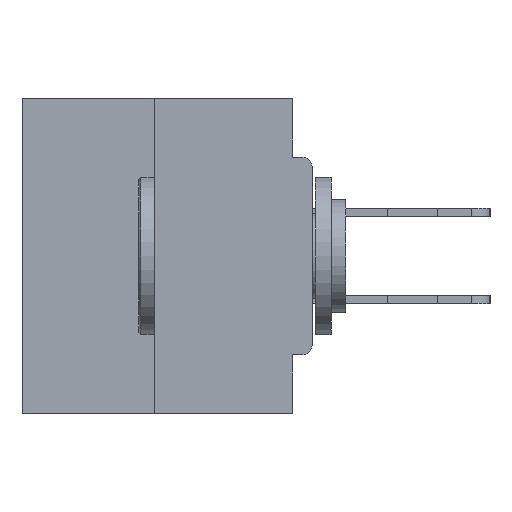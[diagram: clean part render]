
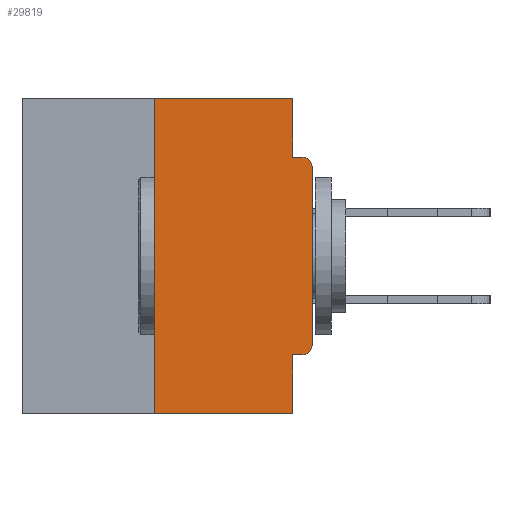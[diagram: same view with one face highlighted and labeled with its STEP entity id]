
A CAD part, left-side view. The second image highlights one B-rep face of the part: STEP entity #29819.
In plain terms, the highlighted planar face has unit normal (-1, 0, 0).
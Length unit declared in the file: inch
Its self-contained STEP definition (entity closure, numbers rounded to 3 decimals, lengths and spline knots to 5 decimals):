
#971 = CARTESIAN_POINT ( 'NONE',  ( 0., 0., -0.4065 ) ) ;
#1369 = DIRECTION ( 'NONE',  ( 0., -1., 0. ) ) ;
#1445 = CARTESIAN_POINT ( 'NONE',  ( 0., 0.031, 0. ) ) ;
#1737 = ORIENTED_EDGE ( 'NONE', *, *, #7454, .T. ) ;
#2048 = VERTEX_POINT ( 'NONE', #5673 ) ;
#2219 = ORIENTED_EDGE ( 'NONE', *, *, #28640, .F. ) ;
#2368 = VERTEX_POINT ( 'NONE', #9984 ) ;
#2789 = ORIENTED_EDGE ( 'NONE', *, *, #19677, .F. ) ;
#3756 = AXIS2_PLACEMENT_3D ( 'NONE', #20615, #26298, #30040 ) ;
#3862 = CARTESIAN_POINT ( 'NONE',  ( 0., 0., -0.1085 ) ) ;
#4383 = DIRECTION ( 'NONE',  ( 0., 0., 1. ) ) ;
#4483 = LINE ( 'NONE', #29040, #16997 ) ;
#4510 = CARTESIAN_POINT ( 'NONE',  ( 0., 0.25, 0. ) ) ;
#4665 = EDGE_CURVE ( 'NONE', #15509, #35964, #20862, .T. ) ;
#5628 = FACE_OUTER_BOUND ( 'NONE', #11698, .T. ) ;
#5673 = CARTESIAN_POINT ( 'NONE',  ( 0., 0., -0.3915 ) ) ;
#6299 = CARTESIAN_POINT ( 'NONE',  ( 0., 0.46, -0.5 ) ) ;
#6460 = VECTOR ( 'NONE', #37101, 39.37008 ) ;
#6672 = VECTOR ( 'NONE', #7743, 39.37008 ) ;
#7227 = VECTOR ( 'NONE', #13439, 39.37008 ) ;
#7454 = EDGE_CURVE ( 'NONE', #23525, #2048, #37386, .T. ) ;
#7743 = DIRECTION ( 'NONE',  ( 0., 0., -1. ) ) ;
#8437 = DIRECTION ( 'NONE',  ( 0., 0., 1. ) ) ;
#9984 = CARTESIAN_POINT ( 'NONE',  ( 0., 0.031, -0.0935 ) ) ;
#10361 = CARTESIAN_POINT ( 'NONE',  ( 0., 0., 0. ) ) ;
#10852 = CARTESIAN_POINT ( 'NONE',  ( 0., 0.25, 0. ) ) ;
#11698 = EDGE_LOOP ( 'NONE', ( #30681, #39686, #39822, #2219, #14073, #1737, #27014, #17364, #2789, #34172 ) ) ;
#12053 = CARTESIAN_POINT ( 'NONE',  ( 0., 0.015, -0.4065 ) ) ;
#12684 = VECTOR ( 'NONE', #4383, 39.37008 ) ;
#13153 = EDGE_CURVE ( 'NONE', #15509, #13797, #21371, .T. ) ;
#13439 = DIRECTION ( 'NONE',  ( 0., 1., 0. ) ) ;
#13484 = VERTEX_POINT ( 'NONE', #25833 ) ;
#13797 = VERTEX_POINT ( 'NONE', #20973 ) ;
#14073 = ORIENTED_EDGE ( 'NONE', *, *, #21989, .F. ) ;
#14296 = CIRCLE ( 'NONE', #32299, 0.015 ) ;
#14626 = LINE ( 'NONE', #21185, #17493 ) ;
#15509 = VERTEX_POINT ( 'NONE', #16903 ) ;
#15910 = DIRECTION ( 'NONE',  ( 0., 0., -1. ) ) ;
#16880 = DIRECTION ( 'NONE',  ( 0., 0., -1. ) ) ;
#16903 = CARTESIAN_POINT ( 'NONE',  ( 0., 0.25, -0.5 ) ) ;
#16997 = VECTOR ( 'NONE', #1369, 39.37008 ) ;
#17364 = ORIENTED_EDGE ( 'NONE', *, *, #17976, .T. ) ;
#17387 = VERTEX_POINT ( 'NONE', #19023 ) ;
#17493 = VECTOR ( 'NONE', #33547, 39.37008 ) ;
#17523 = PLANE ( 'NONE',  #3756 ) ;
#17976 = EDGE_CURVE ( 'NONE', #39611, #13484, #14296, .T. ) ;
#18002 = DIRECTION ( 'NONE',  ( -1., 0., 0. ) ) ;
#19023 = CARTESIAN_POINT ( 'NONE',  ( 0., 0.031, -0.4065 ) ) ;
#19677 = EDGE_CURVE ( 'NONE', #2368, #13484, #14626, .T. ) ;
#20615 = CARTESIAN_POINT ( 'NONE',  ( 0., 0.46, 0. ) ) ;
#20807 = EDGE_CURVE ( 'NONE', #35493, #2368, #21239, .T. ) ;
#20862 = LINE ( 'NONE', #4510, #12684 ) ;
#20973 = CARTESIAN_POINT ( 'NONE',  ( 0., 0.031, -0.5 ) ) ;
#21185 = CARTESIAN_POINT ( 'NONE',  ( 0., 0., -0.0935 ) ) ;
#21239 = LINE ( 'NONE', #1445, #39044 ) ;
#21371 = LINE ( 'NONE', #6299, #6460 ) ;
#21989 = EDGE_CURVE ( 'NONE', #23525, #17387, #34658, .T. ) ;
#23525 = VERTEX_POINT ( 'NONE', #12053 ) ;
#24459 = DIRECTION ( 'NONE',  ( 0., 0., -1. ) ) ;
#25574 = EDGE_CURVE ( 'NONE', #35964, #35493, #4483, .T. ) ;
#25615 = VECTOR ( 'NONE', #8437, 39.37008 ) ;
#25833 = CARTESIAN_POINT ( 'NONE',  ( 0., 0.015, -0.0935 ) ) ;
#26298 = DIRECTION ( 'NONE',  ( 1., 0., 0. ) ) ;
#26480 = AXIS2_PLACEMENT_3D ( 'NONE', #27420, #18002, #24459 ) ;
#27014 = ORIENTED_EDGE ( 'NONE', *, *, #34752, .T. ) ;
#27420 = CARTESIAN_POINT ( 'NONE',  ( 0., 0.015, -0.3915 ) ) ;
#28640 = EDGE_CURVE ( 'NONE', #17387, #13797, #32169, .T. ) ;
#29040 = CARTESIAN_POINT ( 'NONE',  ( 0., 0.46, 0. ) ) ;
#29819 = ADVANCED_FACE ( 'NONE', ( #5628 ), #17523, .F. ) ;
#30040 = DIRECTION ( 'NONE',  ( 0., 0., -1. ) ) ;
#30681 = ORIENTED_EDGE ( 'NONE', *, *, #25574, .F. ) ;
#32169 = LINE ( 'NONE', #34930, #6672 ) ;
#32299 = AXIS2_PLACEMENT_3D ( 'NONE', #34298, #34028, #15910 ) ;
#33547 = DIRECTION ( 'NONE',  ( 0., -1., 0. ) ) ;
#34028 = DIRECTION ( 'NONE',  ( -1., 0., 0. ) ) ;
#34172 = ORIENTED_EDGE ( 'NONE', *, *, #20807, .F. ) ;
#34298 = CARTESIAN_POINT ( 'NONE',  ( 0., 0.015, -0.1085 ) ) ;
#34658 = LINE ( 'NONE', #971, #7227 ) ;
#34752 = EDGE_CURVE ( 'NONE', #2048, #39611, #35721, .T. ) ;
#34930 = CARTESIAN_POINT ( 'NONE',  ( 0., 0.031, -0.5 ) ) ;
#35493 = VERTEX_POINT ( 'NONE', #38765 ) ;
#35721 = LINE ( 'NONE', #10361, #25615 ) ;
#35964 = VERTEX_POINT ( 'NONE', #10852 ) ;
#37101 = DIRECTION ( 'NONE',  ( 0., -1., 0. ) ) ;
#37386 = CIRCLE ( 'NONE', #26480, 0.015 ) ;
#38765 = CARTESIAN_POINT ( 'NONE',  ( 0., 0.031, 0. ) ) ;
#39044 = VECTOR ( 'NONE', #16880, 39.37008 ) ;
#39611 = VERTEX_POINT ( 'NONE', #3862 ) ;
#39686 = ORIENTED_EDGE ( 'NONE', *, *, #4665, .F. ) ;
#39822 = ORIENTED_EDGE ( 'NONE', *, *, #13153, .T. ) ;
